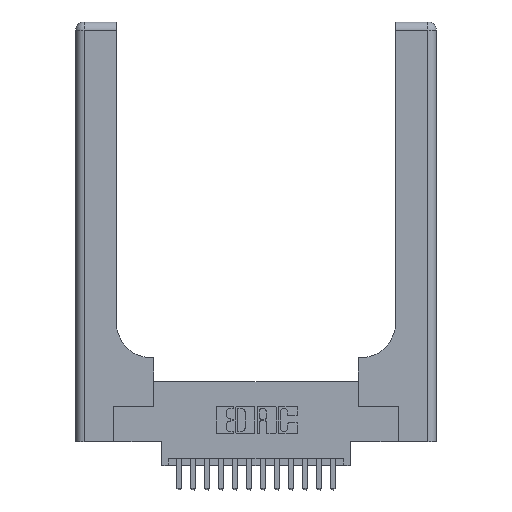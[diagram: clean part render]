
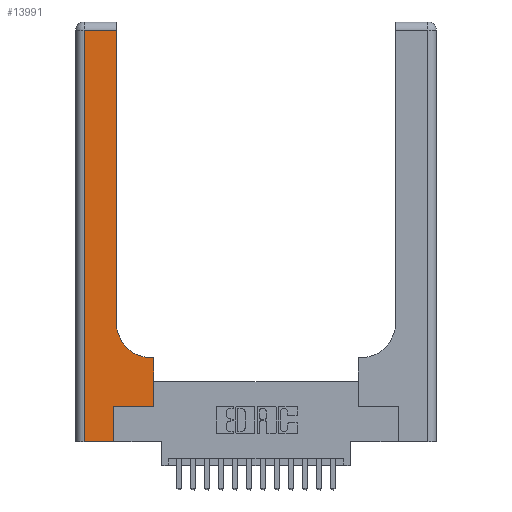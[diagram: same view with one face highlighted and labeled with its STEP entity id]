
A CAD part, top view. The second image highlights one B-rep face of the part: STEP entity #13991.
In plain terms, the highlighted planar face has unit normal (0, 0, 1).
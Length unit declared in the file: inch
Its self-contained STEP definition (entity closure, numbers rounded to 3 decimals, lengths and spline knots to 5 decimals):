
#266 = VECTOR ( 'NONE', #7355, 39.37008 ) ;
#319 = LINE ( 'NONE', #18479, #15404 ) ;
#355 = EDGE_LOOP ( 'NONE', ( #13816, #11162, #18362, #5265, #8776, #5714, #1549, #5964, #17348 ) ) ;
#713 = CARTESIAN_POINT ( 'NONE',  ( 0.5415, 0.6, 0.37 ) ) ;
#728 = LINE ( 'NONE', #5870, #266 ) ;
#1041 = CARTESIAN_POINT ( 'NONE',  ( 0.2915, 0.6, 0.37 ) ) ;
#1202 = DIRECTION ( 'NONE',  ( 0., 1., 0. ) ) ;
#1486 = VECTOR ( 'NONE', #15915, 39.37008 ) ;
#1549 = ORIENTED_EDGE ( 'NONE', *, *, #18590, .T. ) ;
#1830 = PLANE ( 'NONE',  #12187 ) ;
#2023 = AXIS2_PLACEMENT_3D ( 'NONE', #16058, #7413, #17533 ) ;
#2249 = LINE ( 'NONE', #6826, #17263 ) ;
#2393 = CARTESIAN_POINT ( 'NONE',  ( 0.269, 0., 0.37 ) ) ;
#3332 = DIRECTION ( 'NONE',  ( 0., 0., -1. ) ) ;
#3472 = EDGE_CURVE ( 'NONE', #4612, #9269, #2249, .T. ) ;
#3607 = VERTEX_POINT ( 'NONE', #7207 ) ;
#3780 = CARTESIAN_POINT ( 'NONE',  ( 0.5585, 0.6, 0.37 ) ) ;
#4219 = EDGE_CURVE ( 'NONE', #10772, #16682, #5892, .T. ) ;
#4477 = VECTOR ( 'NONE', #1202, 39.37008 ) ;
#4610 = VECTOR ( 'NONE', #12005, 39.37008 ) ;
#4612 = VERTEX_POINT ( 'NONE', #2393 ) ;
#5020 = LINE ( 'NONE', #7739, #12285 ) ;
#5265 = ORIENTED_EDGE ( 'NONE', *, *, #14519, .T. ) ;
#5266 = VERTEX_POINT ( 'NONE', #3780 ) ;
#5416 = DIRECTION ( 'NONE',  ( 0., 1., 0. ) ) ;
#5422 = LINE ( 'NONE', #7188, #1486 ) ;
#5714 = ORIENTED_EDGE ( 'NONE', *, *, #13070, .T. ) ;
#5752 = VERTEX_POINT ( 'NONE', #13967 ) ;
#5779 = CARTESIAN_POINT ( 'NONE',  ( 0.06, 2.94, 0.37 ) ) ;
#5870 = CARTESIAN_POINT ( 'NONE',  ( 0., 2.94, 0.37 ) ) ;
#5892 = CIRCLE ( 'NONE', #2023, 0.25 ) ;
#5964 = ORIENTED_EDGE ( 'NONE', *, *, #10026, .T. ) ;
#6730 = CARTESIAN_POINT ( 'NONE',  ( 0.2915, 0.85, 0.37 ) ) ;
#6826 = CARTESIAN_POINT ( 'NONE',  ( 0.269, 0., 0.37 ) ) ;
#7172 = LINE ( 'NONE', #1041, #8111 ) ;
#7188 = CARTESIAN_POINT ( 'NONE',  ( 0.06, 3., 0.37 ) ) ;
#7207 = CARTESIAN_POINT ( 'NONE',  ( 0.5585, 0.25, 0.37 ) ) ;
#7355 = DIRECTION ( 'NONE',  ( -1., 0., 0. ) ) ;
#7413 = DIRECTION ( 'NONE',  ( 0., 0., -1. ) ) ;
#7661 = EDGE_CURVE ( 'NONE', #9643, #5752, #5422, .T. ) ;
#7739 = CARTESIAN_POINT ( 'NONE',  ( 0.269, 0.25, 0.37 ) ) ;
#8111 = VECTOR ( 'NONE', #11289, 39.37008 ) ;
#8532 = LINE ( 'NONE', #10568, #4610 ) ;
#8776 = ORIENTED_EDGE ( 'NONE', *, *, #3472, .T. ) ;
#9269 = VERTEX_POINT ( 'NONE', #12245 ) ;
#9643 = VERTEX_POINT ( 'NONE', #5779 ) ;
#9979 = CARTESIAN_POINT ( 'NONE',  ( 0.5585, 0.25, 0.37 ) ) ;
#10026 = EDGE_CURVE ( 'NONE', #5266, #10772, #7172, .T. ) ;
#10210 = EDGE_CURVE ( 'NONE', #11578, #9643, #728, .T. ) ;
#10568 = CARTESIAN_POINT ( 'NONE',  ( 0., 0., 0.37 ) ) ;
#10772 = VERTEX_POINT ( 'NONE', #713 ) ;
#11162 = ORIENTED_EDGE ( 'NONE', *, *, #10210, .T. ) ;
#11289 = DIRECTION ( 'NONE',  ( -1., 0., 0. ) ) ;
#11578 = VERTEX_POINT ( 'NONE', #17198 ) ;
#12005 = DIRECTION ( 'NONE',  ( 1., 0., 0. ) ) ;
#12187 = AXIS2_PLACEMENT_3D ( 'NONE', #13428, #3332, #13496 ) ;
#12245 = CARTESIAN_POINT ( 'NONE',  ( 0.269, 0.25, 0.37 ) ) ;
#12285 = VECTOR ( 'NONE', #16390, 39.37008 ) ;
#12699 = DIRECTION ( 'NONE',  ( 0., 1., 0. ) ) ;
#13070 = EDGE_CURVE ( 'NONE', #9269, #3607, #5020, .T. ) ;
#13428 = CARTESIAN_POINT ( 'NONE',  ( 0., 3., 0.37 ) ) ;
#13496 = DIRECTION ( 'NONE',  ( -1., 0., 0. ) ) ;
#13816 = ORIENTED_EDGE ( 'NONE', *, *, #17892, .T. ) ;
#13967 = CARTESIAN_POINT ( 'NONE',  ( 0.06, 0., 0.37 ) ) ;
#13991 = ADVANCED_FACE ( 'NONE', ( #16200 ), #1830, .F. ) ;
#14519 = EDGE_CURVE ( 'NONE', #5752, #4612, #8532, .T. ) ;
#15404 = VECTOR ( 'NONE', #12699, 39.37008 ) ;
#15614 = LINE ( 'NONE', #9979, #4477 ) ;
#15915 = DIRECTION ( 'NONE',  ( 0., -1., 0. ) ) ;
#16058 = CARTESIAN_POINT ( 'NONE',  ( 0.5415, 0.85, 0.37 ) ) ;
#16200 = FACE_OUTER_BOUND ( 'NONE', #355, .T. ) ;
#16390 = DIRECTION ( 'NONE',  ( 1., 0., 0. ) ) ;
#16682 = VERTEX_POINT ( 'NONE', #6730 ) ;
#17198 = CARTESIAN_POINT ( 'NONE',  ( 0.2915, 2.94, 0.37 ) ) ;
#17263 = VECTOR ( 'NONE', #5416, 39.37008 ) ;
#17348 = ORIENTED_EDGE ( 'NONE', *, *, #4219, .T. ) ;
#17533 = DIRECTION ( 'NONE',  ( 1., 0., 0. ) ) ;
#17892 = EDGE_CURVE ( 'NONE', #16682, #11578, #319, .T. ) ;
#18362 = ORIENTED_EDGE ( 'NONE', *, *, #7661, .T. ) ;
#18479 = CARTESIAN_POINT ( 'NONE',  ( 0.2915, 3., 0.37 ) ) ;
#18590 = EDGE_CURVE ( 'NONE', #3607, #5266, #15614, .T. ) ;
